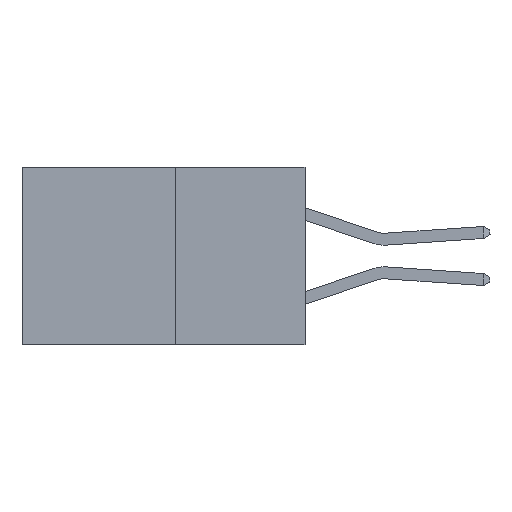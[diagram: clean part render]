
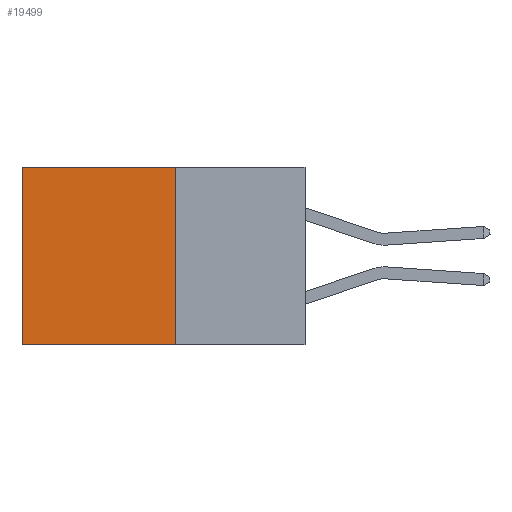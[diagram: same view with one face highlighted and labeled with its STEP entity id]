
A CAD part, left-side view. The second image highlights one B-rep face of the part: STEP entity #19499.
In plain terms, the highlighted planar face has unit normal (-1, 0, 0).
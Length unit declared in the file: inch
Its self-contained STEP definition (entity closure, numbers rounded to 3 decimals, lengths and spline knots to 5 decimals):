
#988 = EDGE_LOOP ( 'NONE', ( #8584, #16805, #25940, #14697 ) ) ;
#2325 = DIRECTION ( 'NONE',  ( 0., 1., 0. ) ) ;
#4056 = LINE ( 'NONE', #17739, #31359 ) ;
#4294 = AXIS2_PLACEMENT_3D ( 'NONE', #14147, #22491, #6135 ) ;
#4605 = CARTESIAN_POINT ( 'NONE',  ( 0.277, 0.27, -0.37 ) ) ;
#6135 = DIRECTION ( 'NONE',  ( 0., 0., -1. ) ) ;
#6185 = VERTEX_POINT ( 'NONE', #17044 ) ;
#6427 = LINE ( 'NONE', #21305, #34516 ) ;
#6756 = EDGE_CURVE ( 'NONE', #22394, #10344, #4056, .T. ) ;
#8584 = ORIENTED_EDGE ( 'NONE', *, *, #6756, .T. ) ;
#9672 = CARTESIAN_POINT ( 'NONE',  ( 0.277, 0.27, 0. ) ) ;
#10014 = FACE_OUTER_BOUND ( 'NONE', #988, .T. ) ;
#10115 = VECTOR ( 'NONE', #18775, 39.37008 ) ;
#10344 = VERTEX_POINT ( 'NONE', #24117 ) ;
#10947 = EDGE_CURVE ( 'NONE', #6185, #10344, #31602, .T. ) ;
#11073 = EDGE_CURVE ( 'NONE', #27618, #22394, #6427, .T. ) ;
#13221 = EDGE_CURVE ( 'NONE', #27618, #6185, #31077, .T. ) ;
#14147 = CARTESIAN_POINT ( 'NONE',  ( 0.277, 0.27, -0.37 ) ) ;
#14697 = ORIENTED_EDGE ( 'NONE', *, *, #11073, .T. ) ;
#16805 = ORIENTED_EDGE ( 'NONE', *, *, #10947, .F. ) ;
#17044 = CARTESIAN_POINT ( 'NONE',  ( 0.277, 0.27, -0.37 ) ) ;
#17178 = DIRECTION ( 'NONE',  ( 0., 0., -1. ) ) ;
#17739 = CARTESIAN_POINT ( 'NONE',  ( 0.277, 0.59, -0.37 ) ) ;
#18775 = DIRECTION ( 'NONE',  ( 0., 0., -1. ) ) ;
#19499 = ADVANCED_FACE ( 'NONE', ( #10014 ), #19726, .F. ) ;
#19726 = PLANE ( 'NONE',  #4294 ) ;
#21305 = CARTESIAN_POINT ( 'NONE',  ( 0.277, 0.27, 0. ) ) ;
#22394 = VERTEX_POINT ( 'NONE', #28964 ) ;
#22491 = DIRECTION ( 'NONE',  ( 1., 0., 0. ) ) ;
#23725 = DIRECTION ( 'NONE',  ( 0., 1., 0. ) ) ;
#24117 = CARTESIAN_POINT ( 'NONE',  ( 0.277, 0.59, -0.37 ) ) ;
#25225 = VECTOR ( 'NONE', #23725, 39.37008 ) ;
#25940 = ORIENTED_EDGE ( 'NONE', *, *, #13221, .F. ) ;
#27618 = VERTEX_POINT ( 'NONE', #9672 ) ;
#28964 = CARTESIAN_POINT ( 'NONE',  ( 0.277, 0.59, 0. ) ) ;
#29761 = CARTESIAN_POINT ( 'NONE',  ( 0.277, 0.27, -0.37 ) ) ;
#31077 = LINE ( 'NONE', #29761, #10115 ) ;
#31359 = VECTOR ( 'NONE', #17178, 39.37008 ) ;
#31602 = LINE ( 'NONE', #4605, #25225 ) ;
#34516 = VECTOR ( 'NONE', #2325, 39.37008 ) ;
